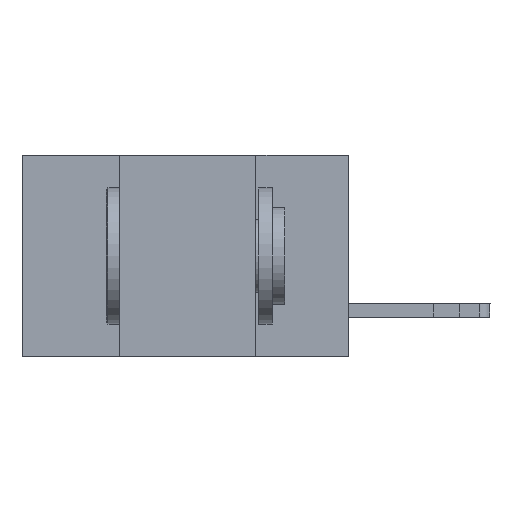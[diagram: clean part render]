
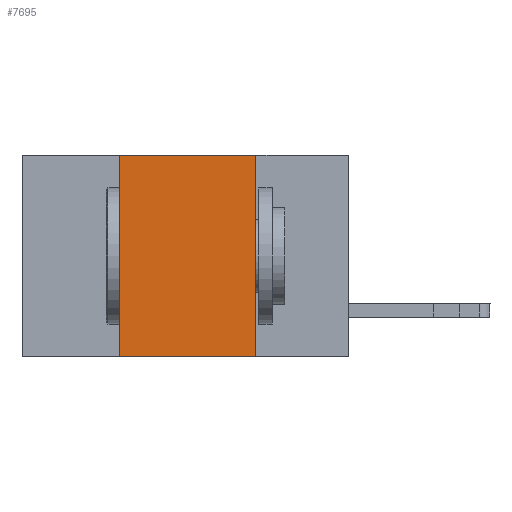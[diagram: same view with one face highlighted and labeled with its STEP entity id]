
A CAD part, left-side view. The second image highlights one B-rep face of the part: STEP entity #7695.
In plain terms, the highlighted planar face has unit normal (-1, 0, 0).
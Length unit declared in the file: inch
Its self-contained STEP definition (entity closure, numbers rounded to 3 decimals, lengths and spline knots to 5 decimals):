
#1597 = CARTESIAN_POINT ( 'NONE',  ( 0., 0.17, 0. ) ) ;
#1695 = DIRECTION ( 'NONE',  ( 0., 0., -1. ) ) ;
#1775 = ORIENTED_EDGE ( 'NONE', *, *, #15122, .F. ) ;
#1796 = CARTESIAN_POINT ( 'NONE',  ( 0., 0.17, -0.37 ) ) ;
#2161 = DIRECTION ( 'NONE',  ( 0., 0., 1. ) ) ;
#2389 = ORIENTED_EDGE ( 'NONE', *, *, #9537, .F. ) ;
#2621 = DIRECTION ( 'NONE',  ( 0., -1., 0. ) ) ;
#2818 = CARTESIAN_POINT ( 'NONE',  ( 0., 0.6, 0. ) ) ;
#2906 = FACE_OUTER_BOUND ( 'NONE', #2909, .T. ) ;
#2909 = EDGE_LOOP ( 'NONE', ( #2389, #18356, #1775, #18299 ) ) ;
#4732 = EDGE_CURVE ( 'NONE', #7132, #12190, #8841, .T. ) ;
#5890 = VECTOR ( 'NONE', #2161, 39.37008 ) ;
#6622 = CARTESIAN_POINT ( 'NONE',  ( 0., 0.42, 0. ) ) ;
#7132 = VERTEX_POINT ( 'NONE', #17968 ) ;
#7695 = ADVANCED_FACE ( 'NONE', ( #2906 ), #16847, .F. ) ;
#7886 = CARTESIAN_POINT ( 'NONE',  ( 0., 0.42, 0. ) ) ;
#8841 = LINE ( 'NONE', #10059, #10294 ) ;
#9273 = DIRECTION ( 'NONE',  ( 0., 0., -1. ) ) ;
#9537 = EDGE_CURVE ( 'NONE', #10025, #12190, #13647, .T. ) ;
#10025 = VERTEX_POINT ( 'NONE', #17197 ) ;
#10059 = CARTESIAN_POINT ( 'NONE',  ( 0., 0.6, -0.37 ) ) ;
#10294 = VECTOR ( 'NONE', #16229, 39.37008 ) ;
#10532 = AXIS2_PLACEMENT_3D ( 'NONE', #2818, #18138, #9273 ) ;
#12190 = VERTEX_POINT ( 'NONE', #1796 ) ;
#13193 = LINE ( 'NONE', #15993, #17023 ) ;
#13647 = LINE ( 'NONE', #1597, #19169 ) ;
#14213 = LINE ( 'NONE', #6622, #5890 ) ;
#15122 = EDGE_CURVE ( 'NONE', #7132, #15400, #14213, .T. ) ;
#15234 = EDGE_CURVE ( 'NONE', #15400, #10025, #13193, .T. ) ;
#15400 = VERTEX_POINT ( 'NONE', #7886 ) ;
#15993 = CARTESIAN_POINT ( 'NONE',  ( 0., 0.6, 0. ) ) ;
#16229 = DIRECTION ( 'NONE',  ( 0., -1., 0. ) ) ;
#16847 = PLANE ( 'NONE',  #10532 ) ;
#17023 = VECTOR ( 'NONE', #2621, 39.37008 ) ;
#17197 = CARTESIAN_POINT ( 'NONE',  ( 0., 0.17, 0. ) ) ;
#17968 = CARTESIAN_POINT ( 'NONE',  ( 0., 0.42, -0.37 ) ) ;
#18138 = DIRECTION ( 'NONE',  ( 1., 0., 0. ) ) ;
#18299 = ORIENTED_EDGE ( 'NONE', *, *, #4732, .T. ) ;
#18356 = ORIENTED_EDGE ( 'NONE', *, *, #15234, .F. ) ;
#19169 = VECTOR ( 'NONE', #1695, 39.37008 ) ;
